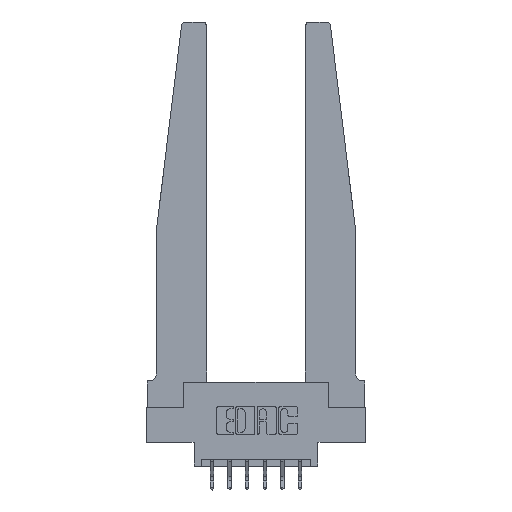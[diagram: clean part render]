
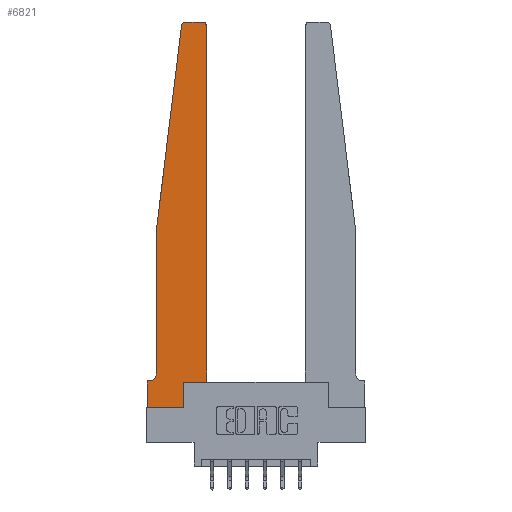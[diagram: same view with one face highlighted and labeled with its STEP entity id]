
A CAD part, top view. The second image highlights one B-rep face of the part: STEP entity #6821.
In plain terms, the highlighted planar face has unit normal (0, 0, 1).
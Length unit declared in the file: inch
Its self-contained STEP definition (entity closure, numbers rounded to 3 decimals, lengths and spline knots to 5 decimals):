
#29 = CARTESIAN_POINT ( 'NONE',  ( 0.2605, 0., 0.37 ) ) ;
#192 = VECTOR ( 'NONE', #5101, 39.37008 ) ;
#276 = DIRECTION ( 'NONE',  ( 0., 0., -1. ) ) ;
#313 = VERTEX_POINT ( 'NONE', #3069 ) ;
#399 = ORIENTED_EDGE ( 'NONE', *, *, #6583, .T. ) ;
#555 = DIRECTION ( 'NONE',  ( 0., 1., 0. ) ) ;
#611 = VERTEX_POINT ( 'NONE', #2639 ) ;
#703 = PLANE ( 'NONE',  #1083 ) ;
#1083 = AXIS2_PLACEMENT_3D ( 'NONE', #11385, #1786, #9308 ) ;
#1120 = VECTOR ( 'NONE', #2203, 39.37008 ) ;
#1156 = CARTESIAN_POINT ( 'NONE',  ( 0., 0., 0.37 ) ) ;
#1537 = AXIS2_PLACEMENT_3D ( 'NONE', #12035, #5639, #13105 ) ;
#1674 = CARTESIAN_POINT ( 'NONE',  ( 0.2605, 0.18, 0.37 ) ) ;
#1756 = VECTOR ( 'NONE', #5392, 39.37008 ) ;
#1786 = DIRECTION ( 'NONE',  ( 0., 0., 1. ) ) ;
#1823 = EDGE_CURVE ( 'NONE', #7359, #7555, #5595, .T. ) ;
#2150 = VERTEX_POINT ( 'NONE', #10974 ) ;
#2203 = DIRECTION ( 'NONE',  ( 1., 0., 0. ) ) ;
#2205 = VECTOR ( 'NONE', #5039, 39.37008 ) ;
#2286 = ORIENTED_EDGE ( 'NONE', *, *, #10555, .T. ) ;
#2297 = ORIENTED_EDGE ( 'NONE', *, *, #6794, .T. ) ;
#2368 = DIRECTION ( 'NONE',  ( -1., 0., 0. ) ) ;
#2481 = EDGE_CURVE ( 'NONE', #611, #10019, #9264, .T. ) ;
#2560 = EDGE_CURVE ( 'NONE', #10443, #7530, #5406, .T. ) ;
#2639 = CARTESIAN_POINT ( 'NONE',  ( 0.27653, 2.75, 0.37 ) ) ;
#2644 = EDGE_CURVE ( 'NONE', #7530, #4869, #5070, .T. ) ;
#2757 = VECTOR ( 'NONE', #8166, 39.37008 ) ;
#2842 = ORIENTED_EDGE ( 'NONE', *, *, #2481, .T. ) ;
#2845 = CARTESIAN_POINT ( 'NONE',  ( 0.24675, 2.72367, 0.37 ) ) ;
#2888 = CARTESIAN_POINT ( 'NONE',  ( 0.425, 0.18, 0.37 ) ) ;
#3069 = CARTESIAN_POINT ( 'NONE',  ( 0., 0., 0.37 ) ) ;
#3095 = CARTESIAN_POINT ( 'NONE',  ( 0.015, 0.1875, 0.37 ) ) ;
#3451 = CARTESIAN_POINT ( 'NONE',  ( 0., 0., 0.37 ) ) ;
#3799 = CARTESIAN_POINT ( 'NONE',  ( 0.425, 0.18, 0.37 ) ) ;
#3872 = ORIENTED_EDGE ( 'NONE', *, *, #10691, .T. ) ;
#4349 = ORIENTED_EDGE ( 'NONE', *, *, #2560, .T. ) ;
#4503 = ORIENTED_EDGE ( 'NONE', *, *, #1823, .T. ) ;
#4525 = DIRECTION ( 'NONE',  ( 0., -1., 0. ) ) ;
#4754 = EDGE_CURVE ( 'NONE', #8330, #2150, #12165, .T. ) ;
#4855 = AXIS2_PLACEMENT_3D ( 'NONE', #5846, #13312, #6901 ) ;
#4869 = VERTEX_POINT ( 'NONE', #3799 ) ;
#5039 = DIRECTION ( 'NONE',  ( 1., 0., 0. ) ) ;
#5070 = LINE ( 'NONE', #2888, #2205 ) ;
#5101 = DIRECTION ( 'NONE',  ( -1., 0., 0. ) ) ;
#5316 = VERTEX_POINT ( 'NONE', #6387 ) ;
#5392 = DIRECTION ( 'NONE',  ( 0., -1., 0. ) ) ;
#5406 = LINE ( 'NONE', #8066, #8239 ) ;
#5460 = VECTOR ( 'NONE', #4525, 39.37008 ) ;
#5595 = LINE ( 'NONE', #12333, #192 ) ;
#5616 = LINE ( 'NONE', #6032, #2757 ) ;
#5639 = DIRECTION ( 'NONE',  ( 0., 0., 1. ) ) ;
#5758 = VERTEX_POINT ( 'NONE', #8518 ) ;
#5846 = CARTESIAN_POINT ( 'NONE',  ( 0.27653, 2.72, 0.37 ) ) ;
#6032 = CARTESIAN_POINT ( 'NONE',  ( 0.065, 1.25, 0.37 ) ) ;
#6125 = LINE ( 'NONE', #6681, #7943 ) ;
#6262 = AXIS2_PLACEMENT_3D ( 'NONE', #6718, #276, #7783 ) ;
#6387 = CARTESIAN_POINT ( 'NONE',  ( 0.065, 0.2375, 0.37 ) ) ;
#6558 = EDGE_CURVE ( 'NONE', #7555, #313, #11135, .T. ) ;
#6574 = ORIENTED_EDGE ( 'NONE', *, *, #4754, .T. ) ;
#6583 = EDGE_CURVE ( 'NONE', #2150, #611, #6125, .T. ) ;
#6681 = CARTESIAN_POINT ( 'NONE',  ( 0.25, 2.75, 0.37 ) ) ;
#6718 = CARTESIAN_POINT ( 'NONE',  ( 0.015, 0.2375, 0.37 ) ) ;
#6794 = EDGE_CURVE ( 'NONE', #10019, #5758, #5616, .T. ) ;
#6821 = ADVANCED_FACE ( 'NONE', ( #10958 ), #703, .T. ) ;
#6865 = ORIENTED_EDGE ( 'NONE', *, *, #2644, .T. ) ;
#6901 = DIRECTION ( 'NONE',  ( 1., 0., 0. ) ) ;
#7359 = VERTEX_POINT ( 'NONE', #3095 ) ;
#7485 = ORIENTED_EDGE ( 'NONE', *, *, #13767, .T. ) ;
#7530 = VERTEX_POINT ( 'NONE', #1674 ) ;
#7555 = VERTEX_POINT ( 'NONE', #10335 ) ;
#7783 = DIRECTION ( 'NONE',  ( -1., 0., 0. ) ) ;
#7943 = VECTOR ( 'NONE', #2368, 39.37008 ) ;
#8066 = CARTESIAN_POINT ( 'NONE',  ( 0.2605, 0.18, 0.37 ) ) ;
#8166 = DIRECTION ( 'NONE',  ( -0.122, -0.992, 0. ) ) ;
#8239 = VECTOR ( 'NONE', #555, 39.37008 ) ;
#8330 = VERTEX_POINT ( 'NONE', #9709 ) ;
#8518 = CARTESIAN_POINT ( 'NONE',  ( 0.065, 1.25, 0.37 ) ) ;
#9264 = CIRCLE ( 'NONE', #4855, 0.03 ) ;
#9308 = DIRECTION ( 'NONE',  ( 1., 0., 0. ) ) ;
#9709 = CARTESIAN_POINT ( 'NONE',  ( 0.425, 2.72, 0.37 ) ) ;
#9851 = ORIENTED_EDGE ( 'NONE', *, *, #11035, .T. ) ;
#10019 = VERTEX_POINT ( 'NONE', #2845 ) ;
#10201 = LINE ( 'NONE', #12235, #13040 ) ;
#10335 = CARTESIAN_POINT ( 'NONE',  ( 0., 0.1875, 0.37 ) ) ;
#10443 = VERTEX_POINT ( 'NONE', #29 ) ;
#10555 = EDGE_CURVE ( 'NONE', #5316, #7359, #12213, .T. ) ;
#10691 = EDGE_CURVE ( 'NONE', #4869, #8330, #10201, .T. ) ;
#10871 = ORIENTED_EDGE ( 'NONE', *, *, #6558, .T. ) ;
#10902 = EDGE_LOOP ( 'NONE', ( #399, #2842, #2297, #7485, #2286, #4503, #10871, #9851, #4349, #6865, #3872, #6574 ) ) ;
#10958 = FACE_OUTER_BOUND ( 'NONE', #10902, .T. ) ;
#10974 = CARTESIAN_POINT ( 'NONE',  ( 0.395, 2.75, 0.37 ) ) ;
#11035 = EDGE_CURVE ( 'NONE', #313, #10443, #11859, .T. ) ;
#11135 = LINE ( 'NONE', #3451, #5460 ) ;
#11385 = CARTESIAN_POINT ( 'NONE',  ( 0., 0.1875, 0.37 ) ) ;
#11859 = LINE ( 'NONE', #1156, #1120 ) ;
#12035 = CARTESIAN_POINT ( 'NONE',  ( 0.395, 2.72, 0.37 ) ) ;
#12165 = CIRCLE ( 'NONE', #1537, 0.03 ) ;
#12213 = CIRCLE ( 'NONE', #6262, 0.05 ) ;
#12235 = CARTESIAN_POINT ( 'NONE',  ( 0.425, 0.18, 0.37 ) ) ;
#12333 = CARTESIAN_POINT ( 'NONE',  ( 0.065, 0.1875, 0.37 ) ) ;
#12817 = LINE ( 'NONE', #13909, #1756 ) ;
#13040 = VECTOR ( 'NONE', #13310, 39.37008 ) ;
#13105 = DIRECTION ( 'NONE',  ( 1., 0., 0. ) ) ;
#13310 = DIRECTION ( 'NONE',  ( 0., 1., 0. ) ) ;
#13312 = DIRECTION ( 'NONE',  ( 0., 0., 1. ) ) ;
#13767 = EDGE_CURVE ( 'NONE', #5758, #5316, #12817, .T. ) ;
#13909 = CARTESIAN_POINT ( 'NONE',  ( 0.065, 1.25, 0.37 ) ) ;
